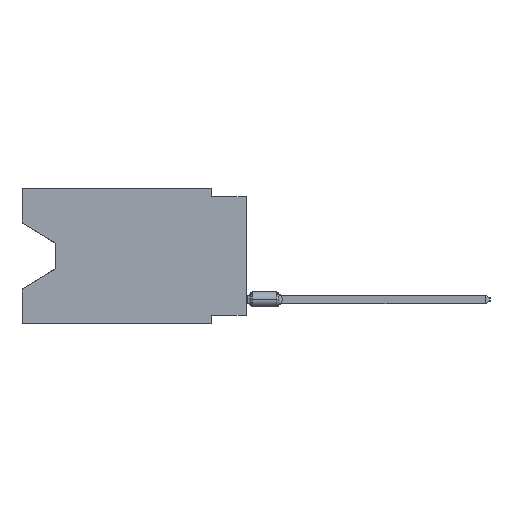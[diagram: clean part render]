
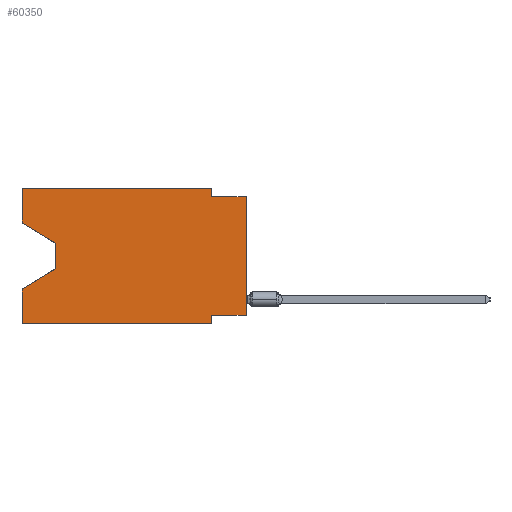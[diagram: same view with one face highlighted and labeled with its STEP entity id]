
A CAD part, left-side view. The second image highlights one B-rep face of the part: STEP entity #60350.
In plain terms, the highlighted planar face has unit normal (-1, 0, 0).
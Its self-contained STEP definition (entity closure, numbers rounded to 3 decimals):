
#1096 = CARTESIAN_POINT ( 'NONE',  ( 0., 16.383, -9.906 ) ) ;
#2103 = ORIENTED_EDGE ( 'NONE', *, *, #35323, .F. ) ;
#3064 = VECTOR ( 'NONE', #75912, 1000. ) ;
#3661 = LINE ( 'NONE', #15981, #13716 ) ;
#3826 = DIRECTION ( 'NONE',  ( 0., 0., 1. ) ) ;
#4673 = EDGE_CURVE ( 'NONE', #30894, #28152, #11647, .T. ) ;
#4752 = ORIENTED_EDGE ( 'NONE', *, *, #4673, .F. ) ;
#5291 = CARTESIAN_POINT ( 'NONE',  ( 0., 13.97, -5.893 ) ) ;
#6709 = CARTESIAN_POINT ( 'NONE',  ( 0., 0., -9.271 ) ) ;
#6846 = CARTESIAN_POINT ( 'NONE',  ( 0., 0., 0. ) ) ;
#7453 = EDGE_CURVE ( 'NONE', #45993, #76294, #19009, .T. ) ;
#7509 = CARTESIAN_POINT ( 'NONE',  ( 0., 16.383, 0. ) ) ;
#10666 = VECTOR ( 'NONE', #80900, 1000. ) ;
#11579 = VECTOR ( 'NONE', #45914, 1000. ) ;
#11647 = LINE ( 'NONE', #37128, #55206 ) ;
#12124 = EDGE_CURVE ( 'NONE', #44660, #16430, #33397, .T. ) ;
#13668 = CARTESIAN_POINT ( 'NONE',  ( 0., 16.383, -2.546 ) ) ;
#13716 = VECTOR ( 'NONE', #48030, 1000. ) ;
#14071 = DIRECTION ( 'NONE',  ( 0., -0.855, -0.519 ) ) ;
#15349 = CARTESIAN_POINT ( 'NONE',  ( 0., 16.383, 0. ) ) ;
#15671 = FACE_OUTER_BOUND ( 'NONE', #51448, .T. ) ;
#15981 = CARTESIAN_POINT ( 'NONE',  ( 0., 16.383, 0. ) ) ;
#15982 = EDGE_CURVE ( 'NONE', #61362, #76294, #43915, .T. ) ;
#16430 = VERTEX_POINT ( 'NONE', #24503 ) ;
#16532 = CARTESIAN_POINT ( 'NONE',  ( 0., 0., -9.271 ) ) ;
#17116 = VERTEX_POINT ( 'NONE', #48453 ) ;
#17543 = CARTESIAN_POINT ( 'NONE',  ( 0., 16.383, -2.546 ) ) ;
#18867 = ORIENTED_EDGE ( 'NONE', *, *, #72534, .F. ) ;
#19009 = LINE ( 'NONE', #7509, #69158 ) ;
#20115 = CARTESIAN_POINT ( 'NONE',  ( 0., 2.54, 0. ) ) ;
#20369 = LINE ( 'NONE', #6846, #3064 ) ;
#20399 = CARTESIAN_POINT ( 'NONE',  ( 0., 16.383, -7.36 ) ) ;
#20817 = VECTOR ( 'NONE', #14071, 1000. ) ;
#22236 = CARTESIAN_POINT ( 'NONE',  ( 0., 16.383, 0. ) ) ;
#24503 = CARTESIAN_POINT ( 'NONE',  ( 0., 13.97, -4.013 ) ) ;
#27027 = LINE ( 'NONE', #46333, #11579 ) ;
#27121 = DIRECTION ( 'NONE',  ( 0., 0., -1. ) ) ;
#27284 = LINE ( 'NONE', #15349, #33687 ) ;
#28152 = VERTEX_POINT ( 'NONE', #63612 ) ;
#29458 = EDGE_CURVE ( 'NONE', #57893, #30894, #46015, .T. ) ;
#30471 = ORIENTED_EDGE ( 'NONE', *, *, #29458, .F. ) ;
#30894 = VERTEX_POINT ( 'NONE', #54047 ) ;
#31564 = DIRECTION ( 'NONE',  ( 0., 0.855, -0.519 ) ) ;
#31809 = ORIENTED_EDGE ( 'NONE', *, *, #55048, .T. ) ;
#31914 = EDGE_CURVE ( 'NONE', #56918, #28152, #20369, .T. ) ;
#33397 = LINE ( 'NONE', #13668, #20817 ) ;
#33687 = VECTOR ( 'NONE', #3826, 1000. ) ;
#34638 = DIRECTION ( 'NONE',  ( 0., 1., 0. ) ) ;
#35176 = ORIENTED_EDGE ( 'NONE', *, *, #66559, .T. ) ;
#35323 = EDGE_CURVE ( 'NONE', #44660, #17116, #27284, .T. ) ;
#36266 = VECTOR ( 'NONE', #34638, 1000. ) ;
#36877 = VERTEX_POINT ( 'NONE', #47843 ) ;
#37128 = CARTESIAN_POINT ( 'NONE',  ( 0., 0., -0.635 ) ) ;
#42579 = CARTESIAN_POINT ( 'NONE',  ( 0., 2.54, -9.906 ) ) ;
#43071 = CARTESIAN_POINT ( 'NONE',  ( 0., 13.97, -4.013 ) ) ;
#43379 = DIRECTION ( 'NONE',  ( 0., 0., -1. ) ) ;
#43915 = LINE ( 'NONE', #5291, #75129 ) ;
#44660 = VERTEX_POINT ( 'NONE', #17543 ) ;
#45765 = ORIENTED_EDGE ( 'NONE', *, *, #15982, .T. ) ;
#45914 = DIRECTION ( 'NONE',  ( 0., -1., 0. ) ) ;
#45993 = VERTEX_POINT ( 'NONE', #1096 ) ;
#46015 = LINE ( 'NONE', #20115, #68681 ) ;
#46333 = CARTESIAN_POINT ( 'NONE',  ( 0., 16.383, -9.906 ) ) ;
#46564 = LINE ( 'NONE', #16532, #36266 ) ;
#47843 = CARTESIAN_POINT ( 'NONE',  ( 0., 2.54, -9.906 ) ) ;
#48030 = DIRECTION ( 'NONE',  ( 0., -1., 0. ) ) ;
#48453 = CARTESIAN_POINT ( 'NONE',  ( 0., 16.383, 0. ) ) ;
#49284 = ORIENTED_EDGE ( 'NONE', *, *, #12124, .T. ) ;
#51448 = EDGE_LOOP ( 'NONE', ( #49284, #31809, #45765, #71890, #35176, #18867, #63888, #69647, #4752, #30471, #80137, #2103 ) ) ;
#51985 = EDGE_CURVE ( 'NONE', #17116, #57893, #3661, .T. ) ;
#53092 = PLANE ( 'NONE',  #78058 ) ;
#54047 = CARTESIAN_POINT ( 'NONE',  ( 0., 2.54, -0.635 ) ) ;
#55048 = EDGE_CURVE ( 'NONE', #16430, #61362, #62000, .T. ) ;
#55206 = VECTOR ( 'NONE', #55646, 1000. ) ;
#55646 = DIRECTION ( 'NONE',  ( 0., -1., 0. ) ) ;
#56918 = VERTEX_POINT ( 'NONE', #6709 ) ;
#57893 = VERTEX_POINT ( 'NONE', #58293 ) ;
#58293 = CARTESIAN_POINT ( 'NONE',  ( 0., 2.54, 0. ) ) ;
#60350 = ADVANCED_FACE ( 'NONE', ( #15671 ), #53092, .F. ) ;
#61362 = VERTEX_POINT ( 'NONE', #80712 ) ;
#62000 = LINE ( 'NONE', #43071, #10666 ) ;
#63092 = CARTESIAN_POINT ( 'NONE',  ( 0., 2.54, -9.271 ) ) ;
#63612 = CARTESIAN_POINT ( 'NONE',  ( 0., 0., -0.635 ) ) ;
#63888 = ORIENTED_EDGE ( 'NONE', *, *, #68160, .F. ) ;
#66559 = EDGE_CURVE ( 'NONE', #45993, #36877, #27027, .T. ) ;
#68160 = EDGE_CURVE ( 'NONE', #56918, #78837, #46564, .T. ) ;
#68681 = VECTOR ( 'NONE', #27121, 1000. ) ;
#69158 = VECTOR ( 'NONE', #69196, 1000. ) ;
#69196 = DIRECTION ( 'NONE',  ( 0., 0., 1. ) ) ;
#69647 = ORIENTED_EDGE ( 'NONE', *, *, #31914, .T. ) ;
#70649 = VECTOR ( 'NONE', #43379, 1000. ) ;
#71890 = ORIENTED_EDGE ( 'NONE', *, *, #7453, .F. ) ;
#72534 = EDGE_CURVE ( 'NONE', #78837, #36877, #79593, .T. ) ;
#72832 = DIRECTION ( 'NONE',  ( 0., 0., -1. ) ) ;
#75129 = VECTOR ( 'NONE', #31564, 1000. ) ;
#75912 = DIRECTION ( 'NONE',  ( 0., 0., 1. ) ) ;
#76294 = VERTEX_POINT ( 'NONE', #20399 ) ;
#78058 = AXIS2_PLACEMENT_3D ( 'NONE', #22236, #78194, #72832 ) ;
#78194 = DIRECTION ( 'NONE',  ( 1., 0., 0. ) ) ;
#78837 = VERTEX_POINT ( 'NONE', #63092 ) ;
#79593 = LINE ( 'NONE', #42579, #70649 ) ;
#80137 = ORIENTED_EDGE ( 'NONE', *, *, #51985, .F. ) ;
#80712 = CARTESIAN_POINT ( 'NONE',  ( 0., 13.97, -5.893 ) ) ;
#80900 = DIRECTION ( 'NONE',  ( 0., 0., -1. ) ) ;
